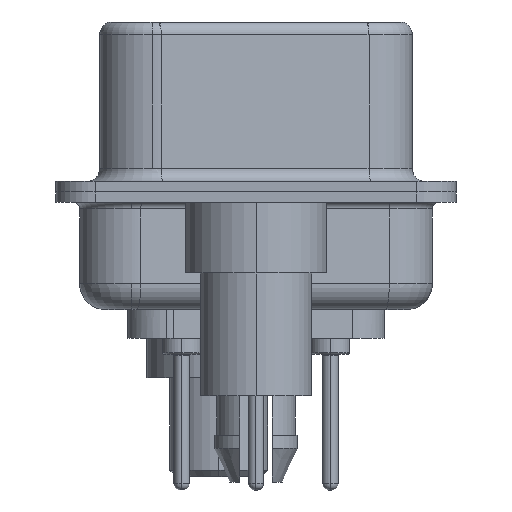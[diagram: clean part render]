
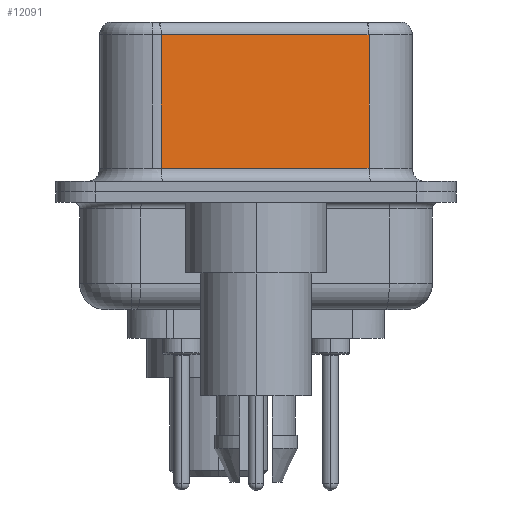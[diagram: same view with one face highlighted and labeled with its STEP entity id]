
A CAD part, left-side view. The second image highlights one B-rep face of the part: STEP entity #12091.
In plain terms, the highlighted planar face has unit normal (-0.985, -0.174, 0).
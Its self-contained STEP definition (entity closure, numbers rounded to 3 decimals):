
#652 = CARTESIAN_POINT ( 'NONE',  ( 3.73, 3.628, 6.52 ) ) ;
#668 = EDGE_CURVE ( 'NONE', #27512, #14980, #1728, .T. ) ;
#1728 = LINE ( 'NONE', #652, #10526 ) ;
#2461 = DIRECTION ( 'NONE',  ( -0.174, 0.985, 0. ) ) ;
#4149 = PLANE ( 'NONE',  #27876 ) ;
#5797 = CARTESIAN_POINT ( 'NONE',  ( 3.73, 3.628, 0.9 ) ) ;
#6066 = DIRECTION ( 'NONE',  ( 0., 0., -1. ) ) ;
#6307 = EDGE_CURVE ( 'NONE', #14980, #28179, #21448, .T. ) ;
#8879 = ORIENTED_EDGE ( 'NONE', *, *, #27398, .T. ) ;
#10034 = EDGE_LOOP ( 'NONE', ( #21041, #8879, #19914, #12921 ) ) ;
#10149 = DIRECTION ( 'NONE',  ( 0.174, -0.985, 0. ) ) ;
#10526 = VECTOR ( 'NONE', #26884, 1000. ) ;
#10745 = VECTOR ( 'NONE', #6066, 1000. ) ;
#11032 = CARTESIAN_POINT ( 'NONE',  ( 5.132, -4.322, 0.9 ) ) ;
#12091 = ADVANCED_FACE ( 'NONE', ( #13414 ), #4149, .F. ) ;
#12921 = ORIENTED_EDGE ( 'NONE', *, *, #6307, .T. ) ;
#13414 = FACE_OUTER_BOUND ( 'NONE', #10034, .T. ) ;
#13671 = LINE ( 'NONE', #16625, #20297 ) ;
#14558 = VERTEX_POINT ( 'NONE', #18005 ) ;
#14980 = VERTEX_POINT ( 'NONE', #5797 ) ;
#15815 = CARTESIAN_POINT ( 'NONE',  ( 5.132, -4.322, 6.52 ) ) ;
#16625 = CARTESIAN_POINT ( 'NONE',  ( 5.132, -4.322, 6.02 ) ) ;
#16828 = CARTESIAN_POINT ( 'NONE',  ( 3.73, 3.628, 6.02 ) ) ;
#16967 = LINE ( 'NONE', #15815, #10745 ) ;
#17643 = DIRECTION ( 'NONE',  ( 0.985, 0.174, 0. ) ) ;
#18005 = CARTESIAN_POINT ( 'NONE',  ( 5.132, -4.322, 6.02 ) ) ;
#19914 = ORIENTED_EDGE ( 'NONE', *, *, #668, .T. ) ;
#20297 = VECTOR ( 'NONE', #2461, 1000. ) ;
#20419 = CARTESIAN_POINT ( 'NONE',  ( 5.132, -4.322, 6.52 ) ) ;
#20715 = VECTOR ( 'NONE', #10149, 1000. ) ;
#21041 = ORIENTED_EDGE ( 'NONE', *, *, #27652, .F. ) ;
#21448 = LINE ( 'NONE', #26140, #20715 ) ;
#26140 = CARTESIAN_POINT ( 'NONE',  ( 5.132, -4.322, 0.9 ) ) ;
#26884 = DIRECTION ( 'NONE',  ( 0., 0., -1. ) ) ;
#27268 = DIRECTION ( 'NONE',  ( -0.174, 0.985, 0. ) ) ;
#27398 = EDGE_CURVE ( 'NONE', #14558, #27512, #13671, .T. ) ;
#27512 = VERTEX_POINT ( 'NONE', #16828 ) ;
#27652 = EDGE_CURVE ( 'NONE', #14558, #28179, #16967, .T. ) ;
#27876 = AXIS2_PLACEMENT_3D ( 'NONE', #20419, #17643, #27268 ) ;
#28179 = VERTEX_POINT ( 'NONE', #11032 ) ;
